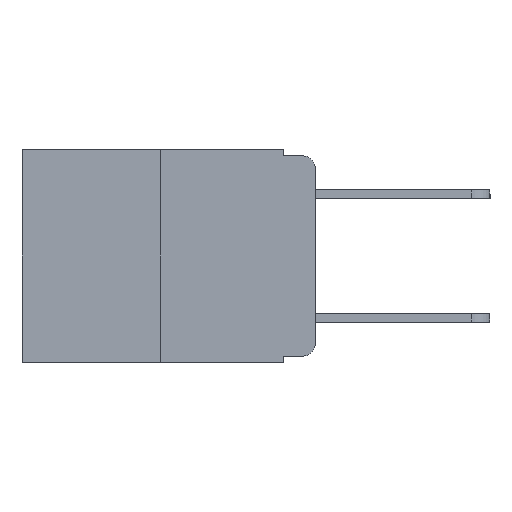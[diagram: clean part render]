
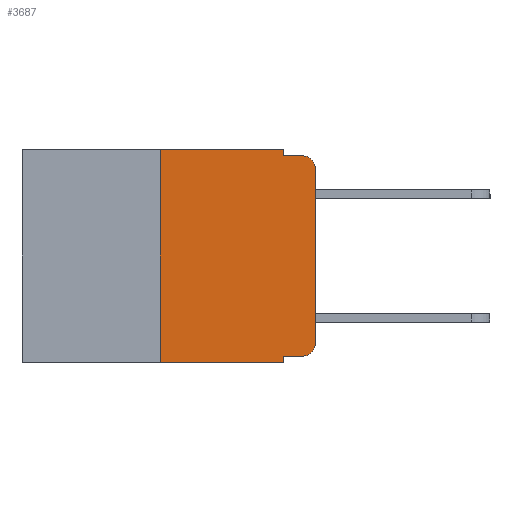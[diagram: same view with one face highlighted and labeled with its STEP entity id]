
A CAD part, left-side view. The second image highlights one B-rep face of the part: STEP entity #3687.
In plain terms, the highlighted planar face has unit normal (-1, 0, 0).
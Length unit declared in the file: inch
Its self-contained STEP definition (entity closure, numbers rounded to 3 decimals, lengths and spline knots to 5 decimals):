
#121 = VERTEX_POINT ( 'NONE', #7600 ) ;
#635 = VECTOR ( 'NONE', #2652, 39.37008 ) ;
#906 = CARTESIAN_POINT ( 'NONE',  ( 0., 0., 0. ) ) ;
#1068 = ORIENTED_EDGE ( 'NONE', *, *, #8067, .F. ) ;
#1254 = VERTEX_POINT ( 'NONE', #5424 ) ;
#1303 = DIRECTION ( 'NONE',  ( 0., 0., -1. ) ) ;
#1536 = CARTESIAN_POINT ( 'NONE',  ( 0., 0.051, -0.333 ) ) ;
#1661 = VECTOR ( 'NONE', #2344, 39.37008 ) ;
#1793 = LINE ( 'NONE', #1536, #4902 ) ;
#1976 = DIRECTION ( 'NONE',  ( 1., 0., 0. ) ) ;
#2192 = ORIENTED_EDGE ( 'NONE', *, *, #8015, .F. ) ;
#2344 = DIRECTION ( 'NONE',  ( 0., -1., 0. ) ) ;
#2540 = VERTEX_POINT ( 'NONE', #14571 ) ;
#2652 = DIRECTION ( 'NONE',  ( 0., -1., 0. ) ) ;
#3687 = ADVANCED_FACE ( 'NONE', ( #9816 ), #16070, .F. ) ;
#3916 = EDGE_LOOP ( 'NONE', ( #5474, #6481, #2192, #9585, #14478, #1068, #6370, #14127, #8737, #5696 ) ) ;
#4046 = DIRECTION ( 'NONE',  ( 0., 0., 1. ) ) ;
#4153 = VECTOR ( 'NONE', #16205, 39.37008 ) ;
#4891 = VERTEX_POINT ( 'NONE', #11233 ) ;
#4902 = VECTOR ( 'NONE', #11542, 39.37008 ) ;
#5424 = CARTESIAN_POINT ( 'NONE',  ( 0., 0.051, -0.343 ) ) ;
#5474 = ORIENTED_EDGE ( 'NONE', *, *, #7943, .T. ) ;
#5477 = DIRECTION ( 'NONE',  ( 0., 0., -1. ) ) ;
#5528 = VERTEX_POINT ( 'NONE', #13679 ) ;
#5584 = DIRECTION ( 'NONE',  ( -1., 0., 0. ) ) ;
#5696 = ORIENTED_EDGE ( 'NONE', *, *, #8120, .T. ) ;
#5906 = CIRCLE ( 'NONE', #7064, 0.02 ) ;
#6090 = LINE ( 'NONE', #12675, #9755 ) ;
#6115 = CARTESIAN_POINT ( 'NONE',  ( 0., 0., -0.313 ) ) ;
#6156 = EDGE_CURVE ( 'NONE', #4891, #12253, #8546, .T. ) ;
#6338 = CARTESIAN_POINT ( 'NONE',  ( 0., 0.02, -0.03 ) ) ;
#6344 = CARTESIAN_POINT ( 'NONE',  ( 0., 0.473, 0. ) ) ;
#6370 = ORIENTED_EDGE ( 'NONE', *, *, #6858, .T. ) ;
#6481 = ORIENTED_EDGE ( 'NONE', *, *, #7971, .T. ) ;
#6617 = CARTESIAN_POINT ( 'NONE',  ( 0., 0.051, 0. ) ) ;
#6858 = EDGE_CURVE ( 'NONE', #13896, #1254, #13871, .T. ) ;
#7064 = AXIS2_PLACEMENT_3D ( 'NONE', #6338, #14747, #7605 ) ;
#7187 = CARTESIAN_POINT ( 'NONE',  ( 0., 0.473, 0. ) ) ;
#7600 = CARTESIAN_POINT ( 'NONE',  ( 0., 0.051, -0.333 ) ) ;
#7605 = DIRECTION ( 'NONE',  ( 0., 0., -1. ) ) ;
#7670 = VECTOR ( 'NONE', #14987, 39.37008 ) ;
#7826 = CARTESIAN_POINT ( 'NONE',  ( 0., 0.051, 0. ) ) ;
#7943 = EDGE_CURVE ( 'NONE', #15098, #11682, #16228, .T. ) ;
#7971 = EDGE_CURVE ( 'NONE', #11682, #15221, #5906, .T. ) ;
#8015 = EDGE_CURVE ( 'NONE', #2540, #15221, #10476, .T. ) ;
#8039 = EDGE_CURVE ( 'NONE', #12253, #2540, #10111, .T. ) ;
#8067 = EDGE_CURVE ( 'NONE', #13896, #4891, #6090, .T. ) ;
#8098 = EDGE_CURVE ( 'NONE', #121, #1254, #14945, .T. ) ;
#8103 = EDGE_CURVE ( 'NONE', #121, #5528, #1793, .T. ) ;
#8120 = EDGE_CURVE ( 'NONE', #5528, #15098, #10953, .T. ) ;
#8546 = LINE ( 'NONE', #6344, #1661 ) ;
#8640 = VECTOR ( 'NONE', #5477, 39.37008 ) ;
#8737 = ORIENTED_EDGE ( 'NONE', *, *, #8103, .T. ) ;
#9249 = AXIS2_PLACEMENT_3D ( 'NONE', #12899, #5584, #14055 ) ;
#9585 = ORIENTED_EDGE ( 'NONE', *, *, #8039, .F. ) ;
#9755 = VECTOR ( 'NONE', #4046, 39.37008 ) ;
#9816 = FACE_OUTER_BOUND ( 'NONE', #3916, .T. ) ;
#10111 = LINE ( 'NONE', #6617, #7670 ) ;
#10151 = CARTESIAN_POINT ( 'NONE',  ( 0., 0.051, -0.01 ) ) ;
#10476 = LINE ( 'NONE', #10151, #635 ) ;
#10953 = CIRCLE ( 'NONE', #9249, 0.02 ) ;
#11007 = DIRECTION ( 'NONE',  ( 0., 0., 1. ) ) ;
#11233 = CARTESIAN_POINT ( 'NONE',  ( 0., 0.25, 0. ) ) ;
#11542 = DIRECTION ( 'NONE',  ( 0., -1., 0. ) ) ;
#11682 = VERTEX_POINT ( 'NONE', #15094 ) ;
#12253 = VERTEX_POINT ( 'NONE', #7826 ) ;
#12645 = AXIS2_PLACEMENT_3D ( 'NONE', #7187, #1976, #1303 ) ;
#12675 = CARTESIAN_POINT ( 'NONE',  ( 0., 0.25, 0. ) ) ;
#12754 = VECTOR ( 'NONE', #11007, 39.37008 ) ;
#12899 = CARTESIAN_POINT ( 'NONE',  ( 0., 0.02, -0.313 ) ) ;
#12998 = CARTESIAN_POINT ( 'NONE',  ( 0., 0.25, -0.343 ) ) ;
#13679 = CARTESIAN_POINT ( 'NONE',  ( 0., 0.02, -0.333 ) ) ;
#13871 = LINE ( 'NONE', #16234, #4153 ) ;
#13896 = VERTEX_POINT ( 'NONE', #12998 ) ;
#13952 = CARTESIAN_POINT ( 'NONE',  ( 0., 0.051, 0. ) ) ;
#14055 = DIRECTION ( 'NONE',  ( 0., 0., -1. ) ) ;
#14127 = ORIENTED_EDGE ( 'NONE', *, *, #8098, .F. ) ;
#14478 = ORIENTED_EDGE ( 'NONE', *, *, #6156, .F. ) ;
#14571 = CARTESIAN_POINT ( 'NONE',  ( 0., 0.051, -0.01 ) ) ;
#14747 = DIRECTION ( 'NONE',  ( -1., 0., 0. ) ) ;
#14945 = LINE ( 'NONE', #13952, #8640 ) ;
#14987 = DIRECTION ( 'NONE',  ( 0., 0., -1. ) ) ;
#15094 = CARTESIAN_POINT ( 'NONE',  ( 0., 0., -0.03 ) ) ;
#15098 = VERTEX_POINT ( 'NONE', #6115 ) ;
#15115 = CARTESIAN_POINT ( 'NONE',  ( 0., 0.02, -0.01 ) ) ;
#15221 = VERTEX_POINT ( 'NONE', #15115 ) ;
#16070 = PLANE ( 'NONE',  #12645 ) ;
#16205 = DIRECTION ( 'NONE',  ( 0., -1., 0. ) ) ;
#16228 = LINE ( 'NONE', #906, #12754 ) ;
#16234 = CARTESIAN_POINT ( 'NONE',  ( 0., 0.473, -0.343 ) ) ;
